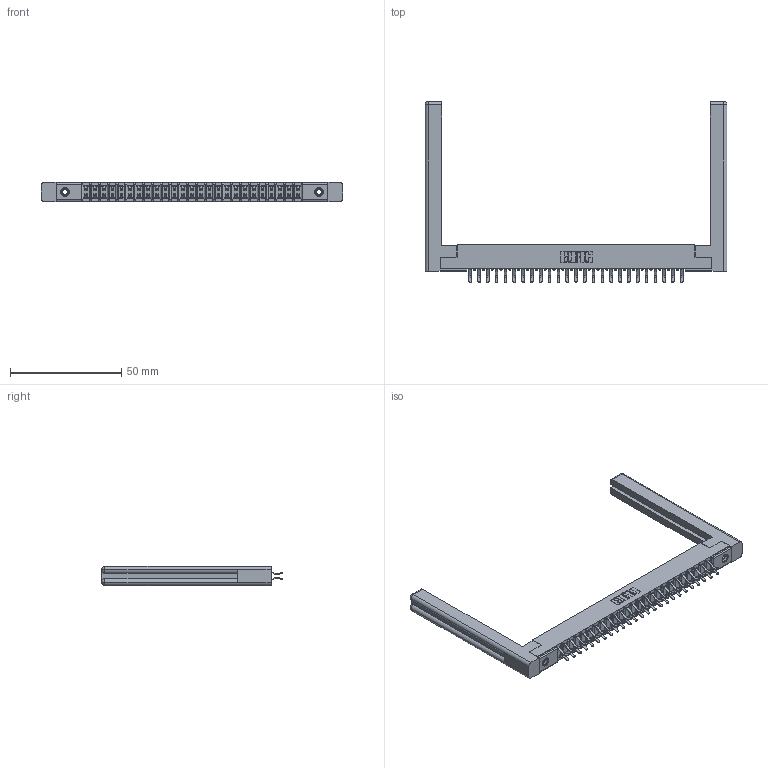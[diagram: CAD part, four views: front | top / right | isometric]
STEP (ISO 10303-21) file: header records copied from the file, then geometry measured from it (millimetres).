
FILE_DESCRIPTION (( 'STEP AP203' ), '1' );
FILE_NAME ('307-050-556-258.STEP', '2019-09-06T11:22:40', ( '' ), ( '' ), 'SwSTEP 2.0', 'SolidWorks 2016', '' );
FILE_SCHEMA (( 'CONFIG_CONTROL_DESIGN' ));
Length unit declared in the file: inch
Products named in the file (5): 307-220-058; 307-290-001_556; 345-250-001_345-250-001-102; 307 Part_.156 Dia Mounting Holes; 307-050-556-258
Assembly tree (55 placements, depth 2):
  307-050-556-258
    307 Part_.156 Dia Mounting Holes
    307-290-001_556  x50
    307-220-058  x2
    345-250-001_345-250-001-102  x2
Bounding box: 135.69 x 81.28 x 8.71 mm (x, y, z)
Volume: 16552.6 mm3; surface area: 20855.4 mm2
Topology: 55 solids, 55 shells, 2786 faces, 7777 edges, 5034 vertices
Faces by surface type: plane 1804, cylinder 906, sphere 52, torus 12, cone 12
Entity records: 27065 total; most frequent: CARTESIAN_POINT 4452, ORIENTED_EDGE 4352, DIRECTION 4326, EDGE_CURVE 2176, LINE 1658, VECTOR 1658, VERTEX_POINT 1406, AXIS2_PLACEMENT_3D 1334
